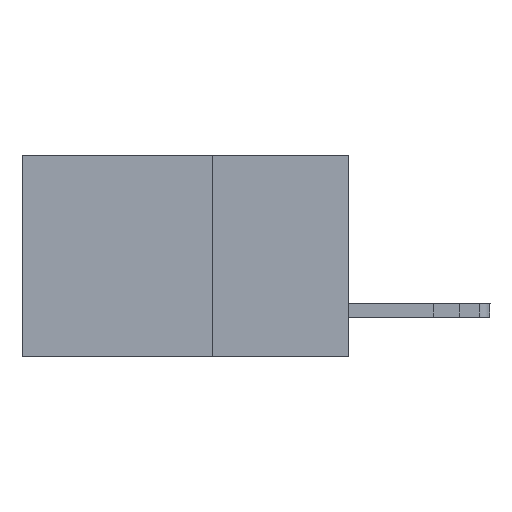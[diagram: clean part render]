
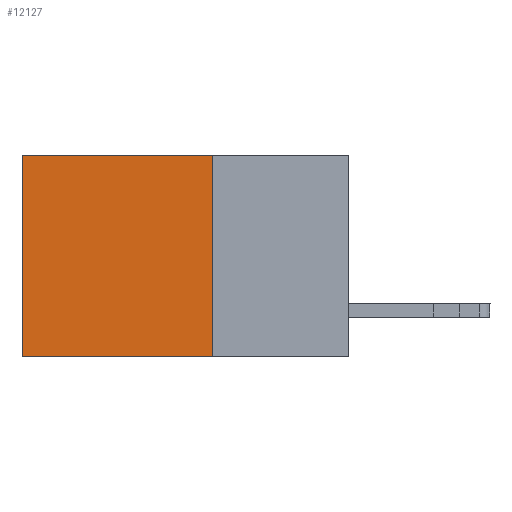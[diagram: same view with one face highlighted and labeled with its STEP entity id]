
A CAD part, left-side view. The second image highlights one B-rep face of the part: STEP entity #12127.
In plain terms, the highlighted planar face has unit normal (-1, 0, 0).
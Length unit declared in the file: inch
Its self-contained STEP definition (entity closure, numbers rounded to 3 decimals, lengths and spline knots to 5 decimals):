
#2 = CARTESIAN_POINT ( 'NONE',  ( 0.298, 0.6, 0. ) ) ;
#237 = CARTESIAN_POINT ( 'NONE',  ( 0.298, 0.25, 0. ) ) ;
#1104 = EDGE_LOOP ( 'NONE', ( #13666, #15790, #10840, #2184 ) ) ;
#1314 = DIRECTION ( 'NONE',  ( 0., 1., 0. ) ) ;
#1559 = EDGE_CURVE ( 'NONE', #4432, #6324, #9595, .T. ) ;
#1773 = CARTESIAN_POINT ( 'NONE',  ( 0.298, 0.6, 0. ) ) ;
#1984 = FACE_OUTER_BOUND ( 'NONE', #1104, .T. ) ;
#2184 = ORIENTED_EDGE ( 'NONE', *, *, #12528, .T. ) ;
#2442 = VERTEX_POINT ( 'NONE', #14522 ) ;
#3360 = DIRECTION ( 'NONE',  ( 0., 1., 0. ) ) ;
#3403 = DIRECTION ( 'NONE',  ( 1., 0., 0. ) ) ;
#3611 = LINE ( 'NONE', #7507, #3654 ) ;
#3654 = VECTOR ( 'NONE', #3360, 39.37008 ) ;
#4432 = VERTEX_POINT ( 'NONE', #237 ) ;
#4545 = CARTESIAN_POINT ( 'NONE',  ( 0.298, 0.25, -0.37 ) ) ;
#5445 = VECTOR ( 'NONE', #1314, 39.37008 ) ;
#5493 = VECTOR ( 'NONE', #13408, 39.37008 ) ;
#5957 = CARTESIAN_POINT ( 'NONE',  ( 0.298, 0.25, 0. ) ) ;
#6104 = LINE ( 'NONE', #15077, #5445 ) ;
#6324 = VERTEX_POINT ( 'NONE', #4545 ) ;
#7336 = AXIS2_PLACEMENT_3D ( 'NONE', #5957, #3403, #12185 ) ;
#7507 = CARTESIAN_POINT ( 'NONE',  ( 0.298, 0.25, 0. ) ) ;
#8863 = LINE ( 'NONE', #2, #12095 ) ;
#9290 = EDGE_CURVE ( 'NONE', #10332, #2442, #8863, .T. ) ;
#9595 = LINE ( 'NONE', #14408, #5493 ) ;
#9701 = PLANE ( 'NONE',  #7336 ) ;
#10108 = DIRECTION ( 'NONE',  ( 0., 0., -1. ) ) ;
#10332 = VERTEX_POINT ( 'NONE', #1773 ) ;
#10840 = ORIENTED_EDGE ( 'NONE', *, *, #1559, .F. ) ;
#12095 = VECTOR ( 'NONE', #10108, 39.37008 ) ;
#12127 = ADVANCED_FACE ( 'NONE', ( #1984 ), #9701, .F. ) ;
#12185 = DIRECTION ( 'NONE',  ( 0., 0., -1. ) ) ;
#12528 = EDGE_CURVE ( 'NONE', #4432, #10332, #3611, .T. ) ;
#13408 = DIRECTION ( 'NONE',  ( 0., 0., -1. ) ) ;
#13666 = ORIENTED_EDGE ( 'NONE', *, *, #9290, .T. ) ;
#14408 = CARTESIAN_POINT ( 'NONE',  ( 0.298, 0.25, 0. ) ) ;
#14522 = CARTESIAN_POINT ( 'NONE',  ( 0.298, 0.6, -0.37 ) ) ;
#15077 = CARTESIAN_POINT ( 'NONE',  ( 0.298, 0.25, -0.37 ) ) ;
#15717 = EDGE_CURVE ( 'NONE', #6324, #2442, #6104, .T. ) ;
#15790 = ORIENTED_EDGE ( 'NONE', *, *, #15717, .F. ) ;
